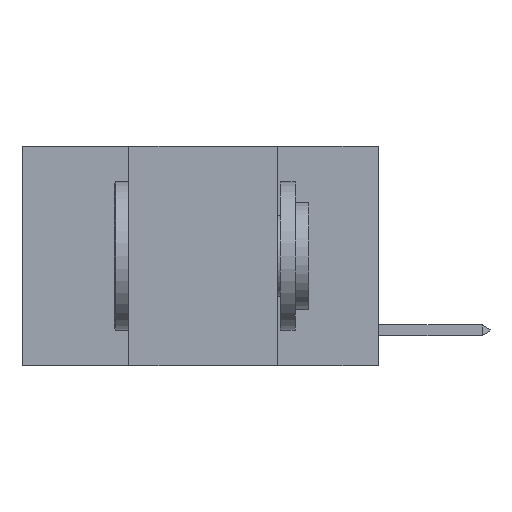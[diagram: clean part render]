
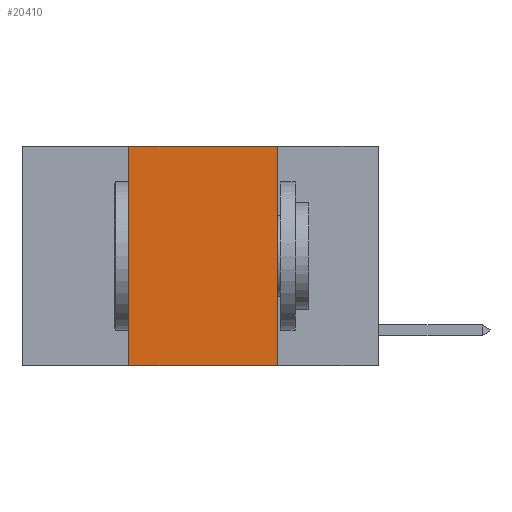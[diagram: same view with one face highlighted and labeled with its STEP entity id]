
A CAD part, left-side view. The second image highlights one B-rep face of the part: STEP entity #20410.
In plain terms, the highlighted planar face has unit normal (-1, 0, 0).
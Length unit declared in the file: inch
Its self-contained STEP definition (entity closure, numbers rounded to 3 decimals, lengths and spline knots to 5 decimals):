
#686 = CARTESIAN_POINT ( 'NONE',  ( 0., 0.17, -0.37 ) ) ;
#1163 = ORIENTED_EDGE ( 'NONE', *, *, #11667, .F. ) ;
#1797 = VECTOR ( 'NONE', #14180, 39.37008 ) ;
#2431 = EDGE_CURVE ( 'NONE', #20203, #10587, #6377, .T. ) ;
#3906 = VERTEX_POINT ( 'NONE', #686 ) ;
#5441 = DIRECTION ( 'NONE',  ( 0., 0., -1. ) ) ;
#6277 = VERTEX_POINT ( 'NONE', #8005 ) ;
#6377 = LINE ( 'NONE', #24177, #18042 ) ;
#7381 = LINE ( 'NONE', #11827, #1797 ) ;
#7891 = CARTESIAN_POINT ( 'NONE',  ( 0., 0.42, 0. ) ) ;
#8005 = CARTESIAN_POINT ( 'NONE',  ( 0., 0.42, -0.37 ) ) ;
#9776 = CARTESIAN_POINT ( 'NONE',  ( 0., 0.6, -0.37 ) ) ;
#10097 = EDGE_CURVE ( 'NONE', #6277, #3906, #29011, .T. ) ;
#10587 = VERTEX_POINT ( 'NONE', #14054 ) ;
#10743 = VECTOR ( 'NONE', #12137, 39.37008 ) ;
#11667 = EDGE_CURVE ( 'NONE', #6277, #20203, #7381, .T. ) ;
#11827 = CARTESIAN_POINT ( 'NONE',  ( 0., 0.42, 0. ) ) ;
#12137 = DIRECTION ( 'NONE',  ( 0., -1., 0. ) ) ;
#12176 = ORIENTED_EDGE ( 'NONE', *, *, #2431, .F. ) ;
#12424 = LINE ( 'NONE', #17168, #17847 ) ;
#12435 = CARTESIAN_POINT ( 'NONE',  ( 0., 0.6, 0. ) ) ;
#12603 = DIRECTION ( 'NONE',  ( 0., 0., -1. ) ) ;
#14054 = CARTESIAN_POINT ( 'NONE',  ( 0., 0.17, 0. ) ) ;
#14180 = DIRECTION ( 'NONE',  ( 0., 0., 1. ) ) ;
#14770 = PLANE ( 'NONE',  #15464 ) ;
#15100 = ORIENTED_EDGE ( 'NONE', *, *, #10097, .T. ) ;
#15464 = AXIS2_PLACEMENT_3D ( 'NONE', #12435, #19434, #5441 ) ;
#16915 = ORIENTED_EDGE ( 'NONE', *, *, #24048, .F. ) ;
#17168 = CARTESIAN_POINT ( 'NONE',  ( 0., 0.17, 0. ) ) ;
#17847 = VECTOR ( 'NONE', #12603, 39.37008 ) ;
#18042 = VECTOR ( 'NONE', #24143, 39.37008 ) ;
#18798 = FACE_OUTER_BOUND ( 'NONE', #18999, .T. ) ;
#18999 = EDGE_LOOP ( 'NONE', ( #16915, #12176, #1163, #15100 ) ) ;
#19434 = DIRECTION ( 'NONE',  ( 1., 0., 0. ) ) ;
#20203 = VERTEX_POINT ( 'NONE', #7891 ) ;
#20410 = ADVANCED_FACE ( 'NONE', ( #18798 ), #14770, .F. ) ;
#24048 = EDGE_CURVE ( 'NONE', #10587, #3906, #12424, .T. ) ;
#24143 = DIRECTION ( 'NONE',  ( 0., -1., 0. ) ) ;
#24177 = CARTESIAN_POINT ( 'NONE',  ( 0., 0.6, 0. ) ) ;
#29011 = LINE ( 'NONE', #9776, #10743 ) ;
